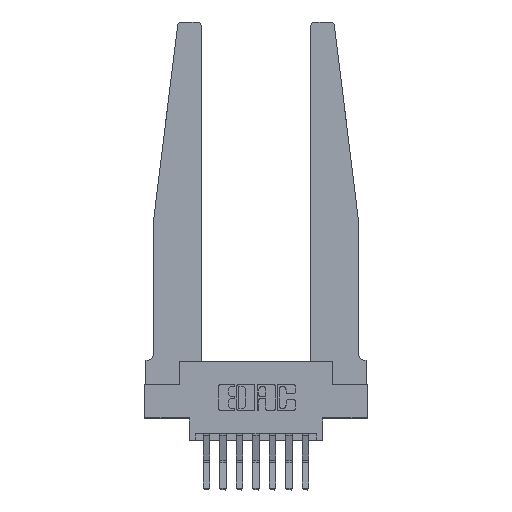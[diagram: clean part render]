
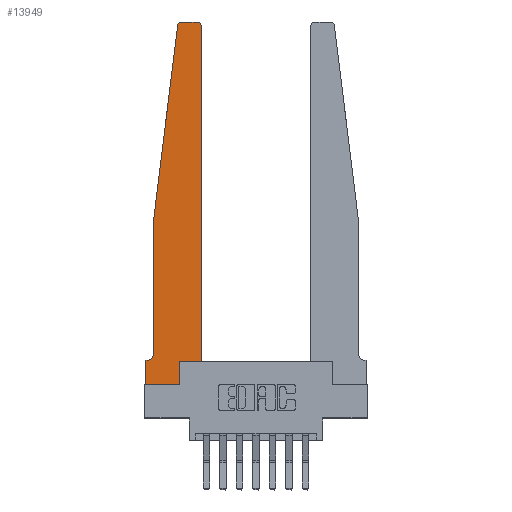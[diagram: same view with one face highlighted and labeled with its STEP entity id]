
A CAD part, top view. The second image highlights one B-rep face of the part: STEP entity #13949.
In plain terms, the highlighted planar face has unit normal (0, 0, 1).
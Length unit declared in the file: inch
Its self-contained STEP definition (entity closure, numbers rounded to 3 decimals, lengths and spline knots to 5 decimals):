
#195 = LINE ( 'NONE', #1155, #465 ) ;
#416 = DIRECTION ( 'NONE',  ( 0., 1., 0. ) ) ;
#465 = VECTOR ( 'NONE', #10106, 39.37008 ) ;
#500 = DIRECTION ( 'NONE',  ( -0.122, -0.992, 0. ) ) ;
#727 = AXIS2_PLACEMENT_3D ( 'NONE', #11926, #13112, #14446 ) ;
#937 = EDGE_CURVE ( 'NONE', #11467, #13280, #12112, .T. ) ;
#1155 = CARTESIAN_POINT ( 'NONE',  ( 0.25, 2.75, 0.37 ) ) ;
#1190 = CARTESIAN_POINT ( 'NONE',  ( 0.015, 0.2375, 0.37 ) ) ;
#1237 = VECTOR ( 'NONE', #13116, 39.37008 ) ;
#2065 = EDGE_CURVE ( 'NONE', #2785, #13447, #9308, .T. ) ;
#2107 = CARTESIAN_POINT ( 'NONE',  ( 0., 0., 0.37 ) ) ;
#2548 = CARTESIAN_POINT ( 'NONE',  ( 0.2605, 0.18, 0.37 ) ) ;
#2584 = CARTESIAN_POINT ( 'NONE',  ( 0.2605, 0., 0.37 ) ) ;
#2596 = CARTESIAN_POINT ( 'NONE',  ( 0.065, 1.25, 0.37 ) ) ;
#2785 = VERTEX_POINT ( 'NONE', #2584 ) ;
#2951 = CARTESIAN_POINT ( 'NONE',  ( 0.065, 0.1875, 0.37 ) ) ;
#3096 = CARTESIAN_POINT ( 'NONE',  ( 0., 0.1875, 0.37 ) ) ;
#3119 = VECTOR ( 'NONE', #10410, 39.37008 ) ;
#3476 = CARTESIAN_POINT ( 'NONE',  ( 0.2605, 0.18, 0.37 ) ) ;
#3673 = CARTESIAN_POINT ( 'NONE',  ( 0., 0., 0.37 ) ) ;
#4064 = DIRECTION ( 'NONE',  ( -1., 0., 0. ) ) ;
#4245 = DIRECTION ( 'NONE',  ( 0., 0., 1. ) ) ;
#4680 = ORIENTED_EDGE ( 'NONE', *, *, #937, .T. ) ;
#4899 = CARTESIAN_POINT ( 'NONE',  ( 0.425, 0.18, 0.37 ) ) ;
#4951 = CARTESIAN_POINT ( 'NONE',  ( 0.425, 0.18, 0.37 ) ) ;
#4995 = FACE_OUTER_BOUND ( 'NONE', #14700, .T. ) ;
#5253 = AXIS2_PLACEMENT_3D ( 'NONE', #1190, #9096, #14662 ) ;
#5323 = VERTEX_POINT ( 'NONE', #8550 ) ;
#5847 = VERTEX_POINT ( 'NONE', #11132 ) ;
#5881 = EDGE_CURVE ( 'NONE', #13614, #6206, #195, .T. ) ;
#5992 = CARTESIAN_POINT ( 'NONE',  ( 0.425, 0.18, 0.37 ) ) ;
#6010 = LINE ( 'NONE', #4899, #9595 ) ;
#6119 = EDGE_CURVE ( 'NONE', #14434, #10559, #14175, .T. ) ;
#6205 = CARTESIAN_POINT ( 'NONE',  ( 0.395, 2.75, 0.37 ) ) ;
#6206 = VERTEX_POINT ( 'NONE', #10979 ) ;
#6343 = DIRECTION ( 'NONE',  ( 1., 0., 0. ) ) ;
#6429 = EDGE_CURVE ( 'NONE', #5847, #13614, #9762, .T. ) ;
#6469 = CARTESIAN_POINT ( 'NONE',  ( 0.065, 1.25, 0.37 ) ) ;
#6476 = PLANE ( 'NONE',  #9547 ) ;
#6590 = EDGE_CURVE ( 'NONE', #5323, #14043, #12148, .T. ) ;
#6744 = ORIENTED_EDGE ( 'NONE', *, *, #7153, .T. ) ;
#7085 = DIRECTION ( 'NONE',  ( 0., 1., 0. ) ) ;
#7153 = EDGE_CURVE ( 'NONE', #13447, #13275, #7421, .T. ) ;
#7376 = ORIENTED_EDGE ( 'NONE', *, *, #6590, .T. ) ;
#7421 = LINE ( 'NONE', #4951, #11194 ) ;
#7608 = EDGE_CURVE ( 'NONE', #10559, #2785, #11038, .T. ) ;
#7805 = ORIENTED_EDGE ( 'NONE', *, *, #6119, .T. ) ;
#7949 = CARTESIAN_POINT ( 'NONE',  ( 0.065, 1.25, 0.37 ) ) ;
#8058 = EDGE_CURVE ( 'NONE', #6206, #11467, #12179, .T. ) ;
#8550 = CARTESIAN_POINT ( 'NONE',  ( 0.065, 0.2375, 0.37 ) ) ;
#8570 = VECTOR ( 'NONE', #12841, 39.37008 ) ;
#8629 = ORIENTED_EDGE ( 'NONE', *, *, #14212, .T. ) ;
#8777 = EDGE_CURVE ( 'NONE', #13275, #5847, #6010, .T. ) ;
#8936 = ORIENTED_EDGE ( 'NONE', *, *, #5881, .T. ) ;
#9096 = DIRECTION ( 'NONE',  ( 0., 0., -1. ) ) ;
#9287 = LINE ( 'NONE', #2596, #3119 ) ;
#9308 = LINE ( 'NONE', #2548, #12944 ) ;
#9387 = ORIENTED_EDGE ( 'NONE', *, *, #2065, .T. ) ;
#9408 = DIRECTION ( 'NONE',  ( 0., 0., 1. ) ) ;
#9473 = DIRECTION ( 'NONE',  ( 1., 0., 0. ) ) ;
#9498 = DIRECTION ( 'NONE',  ( 1., 0., 0. ) ) ;
#9547 = AXIS2_PLACEMENT_3D ( 'NONE', #14427, #9408, #9473 ) ;
#9595 = VECTOR ( 'NONE', #416, 39.37008 ) ;
#9656 = CARTESIAN_POINT ( 'NONE',  ( 0., 0., 0.37 ) ) ;
#9762 = CIRCLE ( 'NONE', #727, 0.03 ) ;
#10106 = DIRECTION ( 'NONE',  ( -1., 0., 0. ) ) ;
#10410 = DIRECTION ( 'NONE',  ( 0., -1., 0. ) ) ;
#10436 = ORIENTED_EDGE ( 'NONE', *, *, #8777, .T. ) ;
#10559 = VERTEX_POINT ( 'NONE', #3673 ) ;
#10887 = ORIENTED_EDGE ( 'NONE', *, *, #8058, .T. ) ;
#10973 = EDGE_CURVE ( 'NONE', #14043, #14434, #13282, .T. ) ;
#10979 = CARTESIAN_POINT ( 'NONE',  ( 0.27653, 2.75, 0.37 ) ) ;
#11038 = LINE ( 'NONE', #2107, #1237 ) ;
#11132 = CARTESIAN_POINT ( 'NONE',  ( 0.425, 2.72, 0.37 ) ) ;
#11194 = VECTOR ( 'NONE', #9498, 39.37008 ) ;
#11246 = VECTOR ( 'NONE', #500, 39.37008 ) ;
#11373 = ORIENTED_EDGE ( 'NONE', *, *, #7608, .T. ) ;
#11467 = VERTEX_POINT ( 'NONE', #11621 ) ;
#11621 = CARTESIAN_POINT ( 'NONE',  ( 0.24675, 2.72367, 0.37 ) ) ;
#11926 = CARTESIAN_POINT ( 'NONE',  ( 0.395, 2.72, 0.37 ) ) ;
#12112 = LINE ( 'NONE', #6469, #11246 ) ;
#12148 = CIRCLE ( 'NONE', #5253, 0.05 ) ;
#12179 = CIRCLE ( 'NONE', #13833, 0.03 ) ;
#12676 = VECTOR ( 'NONE', #4064, 39.37008 ) ;
#12760 = ORIENTED_EDGE ( 'NONE', *, *, #10973, .T. ) ;
#12841 = DIRECTION ( 'NONE',  ( 0., -1., 0. ) ) ;
#12944 = VECTOR ( 'NONE', #7085, 39.37008 ) ;
#13024 = CARTESIAN_POINT ( 'NONE',  ( 0.27653, 2.72, 0.37 ) ) ;
#13112 = DIRECTION ( 'NONE',  ( 0., 0., 1. ) ) ;
#13116 = DIRECTION ( 'NONE',  ( 1., 0., 0. ) ) ;
#13163 = ORIENTED_EDGE ( 'NONE', *, *, #6429, .T. ) ;
#13275 = VERTEX_POINT ( 'NONE', #5992 ) ;
#13280 = VERTEX_POINT ( 'NONE', #7949 ) ;
#13282 = LINE ( 'NONE', #2951, #12676 ) ;
#13447 = VERTEX_POINT ( 'NONE', #3476 ) ;
#13614 = VERTEX_POINT ( 'NONE', #6205 ) ;
#13833 = AXIS2_PLACEMENT_3D ( 'NONE', #13024, #4245, #6343 ) ;
#13949 = ADVANCED_FACE ( 'NONE', ( #4995 ), #6476, .T. ) ;
#14043 = VERTEX_POINT ( 'NONE', #14568 ) ;
#14175 = LINE ( 'NONE', #9656, #8570 ) ;
#14212 = EDGE_CURVE ( 'NONE', #13280, #5323, #9287, .T. ) ;
#14427 = CARTESIAN_POINT ( 'NONE',  ( 0., 0.1875, 0.37 ) ) ;
#14434 = VERTEX_POINT ( 'NONE', #3096 ) ;
#14446 = DIRECTION ( 'NONE',  ( 1., 0., 0. ) ) ;
#14568 = CARTESIAN_POINT ( 'NONE',  ( 0.015, 0.1875, 0.37 ) ) ;
#14662 = DIRECTION ( 'NONE',  ( -1., 0., 0. ) ) ;
#14700 = EDGE_LOOP ( 'NONE', ( #8936, #10887, #4680, #8629, #7376, #12760, #7805, #11373, #9387, #6744, #10436, #13163 ) ) ;
